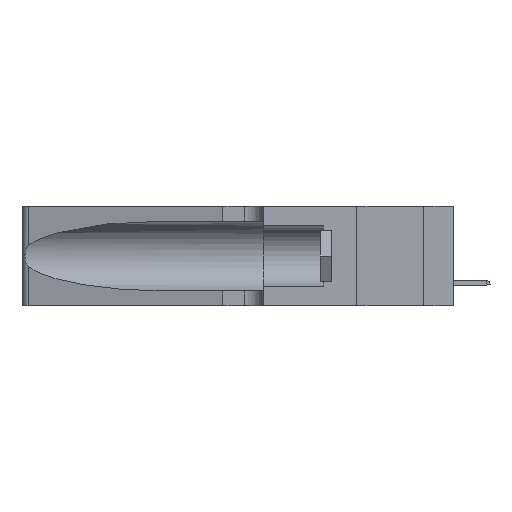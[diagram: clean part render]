
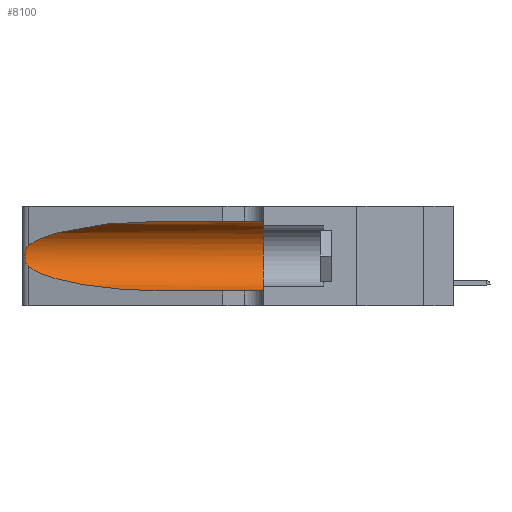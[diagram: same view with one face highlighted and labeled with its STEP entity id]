
A CAD part, left-side view. The second image highlights one B-rep face of the part: STEP entity #8100.
In plain terms, the highlighted cylindrical face has radius 3.308 mm (diameter 6.617 mm), a partial arc.
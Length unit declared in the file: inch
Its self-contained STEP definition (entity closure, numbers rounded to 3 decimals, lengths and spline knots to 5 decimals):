
#1185 = CARTESIAN_POINT ( 'NONE',  ( 0.1305, 0.72297, 0.31525 ) ) ;
#1332 = DIRECTION ( 'NONE',  ( 0., -1., 0. ) ) ;
#2439 = CARTESIAN_POINT ( 'NONE',  ( 0.26075, 1.23896, 0.178 ) ) ;
#3281 = CARTESIAN_POINT ( 'NONE',  ( 0.1305, 0.72297, 0.05475 ) ) ;
#3528 = VERTEX_POINT ( 'NONE', #6105 ) ;
#3653 = FACE_OUTER_BOUND ( 'NONE', #24782, .T. ) ;
#3980 = ORIENTED_EDGE ( 'NONE', *, *, #4949, .F. ) ;
#4643 = EDGE_CURVE ( 'NONE', #7046, #6873, #20139, .T. ) ;
#4706 = CARTESIAN_POINT ( 'NONE',  ( 0.25487, 1.22718, 0.14631 ) ) ;
#4803 = CARTESIAN_POINT ( 'NONE',  ( 0.26017, 1.23833, 0.17102 ) ) ;
#4945 = CARTESIAN_POINT ( 'NONE',  ( 0.25555, 1.22993, 0.14849 ) ) ;
#4949 = EDGE_CURVE ( 'NONE', #17056, #6873, #13481, .T. ) ;
#5092 = ORIENTED_EDGE ( 'NONE', *, *, #16941, .T. ) ;
#6105 = CARTESIAN_POINT ( 'NONE',  ( 0.25487, 1.22718, 0.14631 ) ) ;
#6873 = VERTEX_POINT ( 'NONE', #18024 ) ;
#7046 = VERTEX_POINT ( 'NONE', #3281 ) ;
#7164 = CARTESIAN_POINT ( 'NONE',  ( 0.25856, 1.23593, 0.16098 ) ) ;
#7312 = ORIENTED_EDGE ( 'NONE', *, *, #14721, .T. ) ;
#7771 = CARTESIAN_POINT ( 'NONE',  ( 0.18966, 0.96281, 0.31525 ) ) ;
#8100 = ADVANCED_FACE ( 'NONE', ( #3653 ), #18028, .F. ) ;
#8830 = DIRECTION ( 'NONE',  ( 0., -1., 0. ) ) ;
#8962 = ORIENTED_EDGE ( 'NONE', *, *, #12965, .F. ) ;
#9040 =( BOUNDED_CURVE ( )  B_SPLINE_CURVE ( 3, ( #18651, #7771, #11754, #27602 ),
 .UNSPECIFIED., .F., .F. ) 
 B_SPLINE_CURVE_WITH_KNOTS ( ( 4, 4 ),
 ( 1.5708, 2.84003 ),
 .UNSPECIFIED. ) 
 CURVE ( )  GEOMETRIC_REPRESENTATION_ITEM ( )  RATIONAL_B_SPLINE_CURVE ( ( 1., 0.87, 0.87, 1. ) ) 
 REPRESENTATION_ITEM ( '' )  );
#9362 = CARTESIAN_POINT ( 'NONE',  ( 0.26018, 1.23835, 0.19895 ) ) ;
#10272 = DIRECTION ( 'NONE',  ( 0., 1., 0. ) ) ;
#10288 = DIRECTION ( 'NONE',  ( 0., 0., -1. ) ) ;
#11305 = B_SPLINE_CURVE_WITH_KNOTS ( 'NONE', 3,
 ( #19797, #26556, #11572, #16122, #27416, #9362, #11858, #2439, #4803, #7164, #20811, #25086, #4945, #13628 ),
 .UNSPECIFIED., .F., .F.,
 ( 4, 2, 2, 2, 2, 2, 4 ),
 ( 0., 0.00027, 0.00053, 0.00107, 0.0016, 0.00187, 0.00214 ),
 .UNSPECIFIED. ) ;
#11346 = LINE ( 'NONE', #24722, #21172 ) ;
#11468 = CARTESIAN_POINT ( 'NONE',  ( 0.2373, 1.15595, 0.08982 ) ) ;
#11572 = CARTESIAN_POINT ( 'NONE',  ( 0.25639, 1.23184, 0.21858 ) ) ;
#11754 = CARTESIAN_POINT ( 'NONE',  ( 0.2373, 1.15595, 0.28018 ) ) ;
#11858 = CARTESIAN_POINT ( 'NONE',  ( 0.26075, 1.23896, 0.19203 ) ) ;
#12474 = VERTEX_POINT ( 'NONE', #1185 ) ;
#12965 = EDGE_CURVE ( 'NONE', #12474, #17056, #11346, .T. ) ;
#13272 = VERTEX_POINT ( 'NONE', #17504 ) ;
#13481 = CIRCLE ( 'NONE', #14894, 0.13025 ) ;
#13628 = CARTESIAN_POINT ( 'NONE',  ( 0.25487, 1.22718, 0.14631 ) ) ;
#14721 = EDGE_CURVE ( 'NONE', #3528, #7046, #16004, .T. ) ;
#14894 = AXIS2_PLACEMENT_3D ( 'NONE', #18797, #10272, #26139 ) ;
#16004 =( BOUNDED_CURVE ( )  B_SPLINE_CURVE ( 3, ( #4706, #11468, #18361, #16170 ),
 .UNSPECIFIED., .F., .F. ) 
 B_SPLINE_CURVE_WITH_KNOTS ( ( 4, 4 ),
 ( 3.44316, 4.71239 ),
 .UNSPECIFIED. ) 
 CURVE ( )  GEOMETRIC_REPRESENTATION_ITEM ( )  RATIONAL_B_SPLINE_CURVE ( ( 1., 0.87, 0.87, 1. ) ) 
 REPRESENTATION_ITEM ( '' )  );
#16122 = CARTESIAN_POINT ( 'NONE',  ( 0.25787, 1.23484, 0.2124 ) ) ;
#16170 = CARTESIAN_POINT ( 'NONE',  ( 0.1305, 0.72297, 0.05475 ) ) ;
#16941 = EDGE_CURVE ( 'NONE', #12474, #13272, #9040, .T. ) ;
#17056 = VERTEX_POINT ( 'NONE', #26128 ) ;
#17504 = CARTESIAN_POINT ( 'NONE',  ( 0.25487, 1.22718, 0.22369 ) ) ;
#17657 = CARTESIAN_POINT ( 'NONE',  ( 0.1305, 1.61858, 0.05475 ) ) ;
#18024 = CARTESIAN_POINT ( 'NONE',  ( 0.1305, 0.35, 0.05475 ) ) ;
#18028 = CYLINDRICAL_SURFACE ( 'NONE', #23070, 0.13025 ) ;
#18361 = CARTESIAN_POINT ( 'NONE',  ( 0.18966, 0.96281, 0.05475 ) ) ;
#18623 = VECTOR ( 'NONE', #8830, 39.37008 ) ;
#18651 = CARTESIAN_POINT ( 'NONE',  ( 0.1305, 0.72297, 0.31525 ) ) ;
#18797 = CARTESIAN_POINT ( 'NONE',  ( 0.1305, 0.35, 0.185 ) ) ;
#19797 = CARTESIAN_POINT ( 'NONE',  ( 0.25487, 1.22718, 0.22369 ) ) ;
#20139 = LINE ( 'NONE', #17657, #18623 ) ;
#20311 = DIRECTION ( 'NONE',  ( 0., -1., 0. ) ) ;
#20760 = ORIENTED_EDGE ( 'NONE', *, *, #27577, .T. ) ;
#20811 = CARTESIAN_POINT ( 'NONE',  ( 0.25789, 1.23486, 0.15765 ) ) ;
#21172 = VECTOR ( 'NONE', #20311, 39.37008 ) ;
#22062 = ORIENTED_EDGE ( 'NONE', *, *, #4643, .T. ) ;
#23070 = AXIS2_PLACEMENT_3D ( 'NONE', #23653, #1332, #10288 ) ;
#23653 = CARTESIAN_POINT ( 'NONE',  ( 0.1305, 1.61858, 0.185 ) ) ;
#24722 = CARTESIAN_POINT ( 'NONE',  ( 0.1305, 1.61858, 0.31525 ) ) ;
#24782 = EDGE_LOOP ( 'NONE', ( #5092, #20760, #7312, #22062, #3980, #8962 ) ) ;
#25086 = CARTESIAN_POINT ( 'NONE',  ( 0.25639, 1.23186, 0.15144 ) ) ;
#26128 = CARTESIAN_POINT ( 'NONE',  ( 0.1305, 0.35, 0.31525 ) ) ;
#26139 = DIRECTION ( 'NONE',  ( 0., 0., 1. ) ) ;
#26556 = CARTESIAN_POINT ( 'NONE',  ( 0.25555, 1.22994, 0.2215 ) ) ;
#27416 = CARTESIAN_POINT ( 'NONE',  ( 0.25854, 1.2359, 0.20912 ) ) ;
#27577 = EDGE_CURVE ( 'NONE', #13272, #3528, #11305, .T. ) ;
#27602 = CARTESIAN_POINT ( 'NONE',  ( 0.25487, 1.22718, 0.22369 ) ) ;
